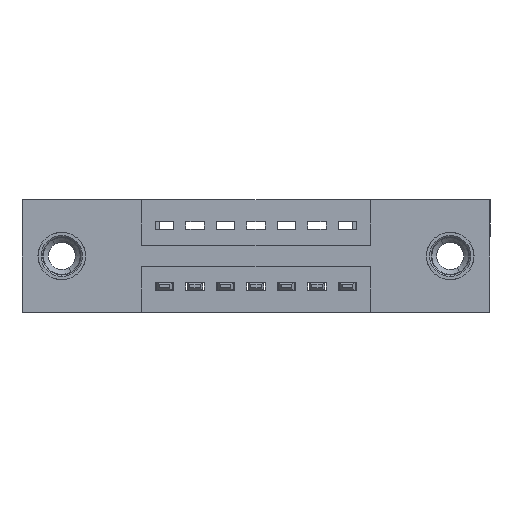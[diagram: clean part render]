
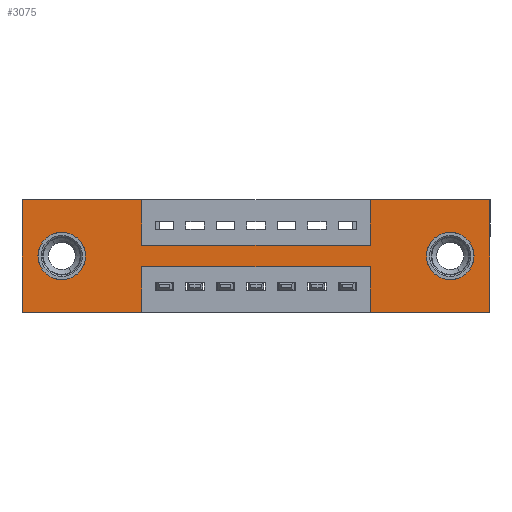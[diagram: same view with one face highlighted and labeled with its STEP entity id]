
A CAD part, front view. The second image highlights one B-rep face of the part: STEP entity #3075.
In plain terms, the highlighted planar face has unit normal (0, -1, 0).
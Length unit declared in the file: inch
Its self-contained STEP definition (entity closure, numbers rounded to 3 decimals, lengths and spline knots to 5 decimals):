
#88 = ORIENTED_EDGE ( 'NONE', *, *, #14354, .F. ) ;
#173 = LINE ( 'NONE', #8126, #4193 ) ;
#216 = DIRECTION ( 'NONE',  ( 1., 0., 0. ) ) ;
#373 = EDGE_CURVE ( 'NONE', #1136, #7667, #10331, .T. ) ;
#400 = DIRECTION ( 'NONE',  ( 0., 0., 1. ) ) ;
#508 = VECTOR ( 'NONE', #2237, 39.37008 ) ;
#535 = ORIENTED_EDGE ( 'NONE', *, *, #14030, .F. ) ;
#603 = CARTESIAN_POINT ( 'NONE',  ( 0.13, 0., -0.107 ) ) ;
#662 = LINE ( 'NONE', #11751, #7004 ) ;
#675 = CIRCLE ( 'NONE', #14537, 0.078 ) ;
#698 = LINE ( 'NONE', #5026, #1076 ) ;
#1076 = VECTOR ( 'NONE', #11715, 39.37008 ) ;
#1115 = VERTEX_POINT ( 'NONE', #603 ) ;
#1120 = VERTEX_POINT ( 'NONE', #5004 ) ;
#1136 = VERTEX_POINT ( 'NONE', #11938 ) ;
#1206 = CARTESIAN_POINT ( 'NONE',  ( 0., 0., -0.37 ) ) ;
#1337 = DIRECTION ( 'NONE',  ( 0., 1., 0. ) ) ;
#1531 = VERTEX_POINT ( 'NONE', #8712 ) ;
#1568 = LINE ( 'NONE', #10457, #3683 ) ;
#1743 = VECTOR ( 'NONE', #14314, 39.37008 ) ;
#1926 = VERTEX_POINT ( 'NONE', #7405 ) ;
#1986 = VECTOR ( 'NONE', #4073, 39.37008 ) ;
#2203 = DIRECTION ( 'NONE',  ( 0., 1., 0. ) ) ;
#2237 = DIRECTION ( 'NONE',  ( 0., 0., 1. ) ) ;
#2255 = ORIENTED_EDGE ( 'NONE', *, *, #14520, .F. ) ;
#2292 = VERTEX_POINT ( 'NONE', #3463 ) ;
#2590 = DIRECTION ( 'NONE',  ( -1., 0., 0. ) ) ;
#2808 = EDGE_LOOP ( 'NONE', ( #3830, #8100 ) ) ;
#2957 = LINE ( 'NONE', #11916, #11040 ) ;
#3075 = ADVANCED_FACE ( 'NONE', ( #6961, #6422, #11164 ), #5661, .T. ) ;
#3146 = EDGE_CURVE ( 'NONE', #7567, #14070, #4483, .T. ) ;
#3203 = EDGE_LOOP ( 'NONE', ( #13448, #6760 ) ) ;
#3404 = AXIS2_PLACEMENT_3D ( 'NONE', #3678, #1337, #400 ) ;
#3463 = CARTESIAN_POINT ( 'NONE',  ( 0.3925, 0., -0.22 ) ) ;
#3465 = DIRECTION ( 'NONE',  ( 0., 0., -1. ) ) ;
#3678 = CARTESIAN_POINT ( 'NONE',  ( 0.13, 0., -0.185 ) ) ;
#3683 = VECTOR ( 'NONE', #4623, 39.37008 ) ;
#3793 = ORIENTED_EDGE ( 'NONE', *, *, #4448, .F. ) ;
#3830 = ORIENTED_EDGE ( 'NONE', *, *, #10777, .T. ) ;
#3854 = CARTESIAN_POINT ( 'NONE',  ( 1.535, 0., -0.37 ) ) ;
#3884 = VERTEX_POINT ( 'NONE', #12785 ) ;
#3994 = DIRECTION ( 'NONE',  ( 0., 0., -1. ) ) ;
#4073 = DIRECTION ( 'NONE',  ( 0., 0., 1. ) ) ;
#4087 = DIRECTION ( 'NONE',  ( 0., 0., 1. ) ) ;
#4193 = VECTOR ( 'NONE', #2590, 39.37008 ) ;
#4389 = ORIENTED_EDGE ( 'NONE', *, *, #5117, .F. ) ;
#4448 = EDGE_CURVE ( 'NONE', #14070, #7242, #4953, .T. ) ;
#4483 = LINE ( 'NONE', #5605, #14157 ) ;
#4623 = DIRECTION ( 'NONE',  ( -1., 0., 0. ) ) ;
#4865 = CIRCLE ( 'NONE', #11131, 0.078 ) ;
#4953 = LINE ( 'NONE', #6335, #1986 ) ;
#5004 = CARTESIAN_POINT ( 'NONE',  ( 0., 0., -0.37 ) ) ;
#5026 = CARTESIAN_POINT ( 'NONE',  ( 0.3925, 0., -0.15 ) ) ;
#5117 = EDGE_CURVE ( 'NONE', #10800, #1926, #5188, .T. ) ;
#5173 = DIRECTION ( 'NONE',  ( 0., 0., 1. ) ) ;
#5188 = LINE ( 'NONE', #11372, #7318 ) ;
#5243 = CARTESIAN_POINT ( 'NONE',  ( 0., 0., 0. ) ) ;
#5605 = CARTESIAN_POINT ( 'NONE',  ( 0., 0., -0.37 ) ) ;
#5608 = VECTOR ( 'NONE', #6076, 39.37008 ) ;
#5661 = PLANE ( 'NONE',  #10589 ) ;
#6037 = CARTESIAN_POINT ( 'NONE',  ( 0.3925, 0., -0.37 ) ) ;
#6076 = DIRECTION ( 'NONE',  ( 0., 0., -1. ) ) ;
#6197 = DIRECTION ( 'NONE',  ( 0., 0., -1. ) ) ;
#6285 = ORIENTED_EDGE ( 'NONE', *, *, #9019, .F. ) ;
#6335 = CARTESIAN_POINT ( 'NONE',  ( 1.1425, 0., -0.37 ) ) ;
#6422 = FACE_BOUND ( 'NONE', #3203, .T. ) ;
#6444 = CARTESIAN_POINT ( 'NONE',  ( 1.1425, 0., -0.37 ) ) ;
#6685 = VECTOR ( 'NONE', #216, 39.37008 ) ;
#6760 = ORIENTED_EDGE ( 'NONE', *, *, #11376, .T. ) ;
#6806 = ORIENTED_EDGE ( 'NONE', *, *, #3146, .F. ) ;
#6824 = ORIENTED_EDGE ( 'NONE', *, *, #11123, .F. ) ;
#6961 = FACE_BOUND ( 'NONE', #2808, .T. ) ;
#7004 = VECTOR ( 'NONE', #6197, 39.37008 ) ;
#7124 = CARTESIAN_POINT ( 'NONE',  ( 1.535, 0., 0. ) ) ;
#7242 = VERTEX_POINT ( 'NONE', #14444 ) ;
#7318 = VECTOR ( 'NONE', #13600, 39.37008 ) ;
#7405 = CARTESIAN_POINT ( 'NONE',  ( 0.3925, 0., -0.15 ) ) ;
#7491 = CARTESIAN_POINT ( 'NONE',  ( 0.3925, 0., 0. ) ) ;
#7567 = VERTEX_POINT ( 'NONE', #3854 ) ;
#7625 = DIRECTION ( 'NONE',  ( 0., 1., 0. ) ) ;
#7667 = VERTEX_POINT ( 'NONE', #11470 ) ;
#7814 = DIRECTION ( 'NONE',  ( 0., -1., 0. ) ) ;
#7921 = CIRCLE ( 'NONE', #10911, 0.078 ) ;
#7998 = CARTESIAN_POINT ( 'NONE',  ( 0., 0., 0. ) ) ;
#8100 = ORIENTED_EDGE ( 'NONE', *, *, #8339, .T. ) ;
#8126 = CARTESIAN_POINT ( 'NONE',  ( 0., 0., -0.37 ) ) ;
#8339 = EDGE_CURVE ( 'NONE', #3884, #9829, #7921, .T. ) ;
#8712 = CARTESIAN_POINT ( 'NONE',  ( 0., 0., 0. ) ) ;
#8922 = EDGE_CURVE ( 'NONE', #1115, #9360, #11775, .T. ) ;
#8928 = ORIENTED_EDGE ( 'NONE', *, *, #14249, .F. ) ;
#9019 = EDGE_CURVE ( 'NONE', #1926, #1136, #698, .T. ) ;
#9246 = DIRECTION ( 'NONE',  ( 0., 1., 0. ) ) ;
#9307 = LINE ( 'NONE', #7998, #6685 ) ;
#9360 = VERTEX_POINT ( 'NONE', #10683 ) ;
#9829 = VERTEX_POINT ( 'NONE', #13728 ) ;
#9953 = VERTEX_POINT ( 'NONE', #6037 ) ;
#10331 = LINE ( 'NONE', #12354, #508 ) ;
#10396 = EDGE_CURVE ( 'NONE', #9953, #1120, #173, .T. ) ;
#10457 = CARTESIAN_POINT ( 'NONE',  ( 0.3925, 0., -0.22 ) ) ;
#10589 = AXIS2_PLACEMENT_3D ( 'NONE', #1206, #7814, #3465 ) ;
#10623 = CARTESIAN_POINT ( 'NONE',  ( 1.535, 0., 0. ) ) ;
#10683 = CARTESIAN_POINT ( 'NONE',  ( 0.13, 0., -0.263 ) ) ;
#10777 = EDGE_CURVE ( 'NONE', #9829, #3884, #675, .T. ) ;
#10800 = VERTEX_POINT ( 'NONE', #7491 ) ;
#10814 = CARTESIAN_POINT ( 'NONE',  ( 1.405, 0., -0.185 ) ) ;
#10911 = AXIS2_PLACEMENT_3D ( 'NONE', #11167, #9246, #12641 ) ;
#11040 = VECTOR ( 'NONE', #5173, 39.37008 ) ;
#11123 = EDGE_CURVE ( 'NONE', #2292, #9953, #662, .T. ) ;
#11131 = AXIS2_PLACEMENT_3D ( 'NONE', #14370, #7625, #4087 ) ;
#11164 = FACE_OUTER_BOUND ( 'NONE', #11595, .T. ) ;
#11167 = CARTESIAN_POINT ( 'NONE',  ( 1.405, 0., -0.185 ) ) ;
#11257 = LINE ( 'NONE', #5243, #1743 ) ;
#11372 = CARTESIAN_POINT ( 'NONE',  ( 0.3925, 0., 0. ) ) ;
#11376 = EDGE_CURVE ( 'NONE', #9360, #1115, #4865, .T. ) ;
#11470 = CARTESIAN_POINT ( 'NONE',  ( 1.1425, 0., 0. ) ) ;
#11595 = EDGE_LOOP ( 'NONE', ( #6824, #11834, #3793, #6806, #88, #8928, #12109, #6285, #4389, #535, #2255, #14294 ) ) ;
#11715 = DIRECTION ( 'NONE',  ( 1., 0., 0. ) ) ;
#11751 = CARTESIAN_POINT ( 'NONE',  ( 0.3925, 0., -0.37 ) ) ;
#11775 = CIRCLE ( 'NONE', #3404, 0.078 ) ;
#11834 = ORIENTED_EDGE ( 'NONE', *, *, #14268, .F. ) ;
#11916 = CARTESIAN_POINT ( 'NONE',  ( 0., 0., 0. ) ) ;
#11938 = CARTESIAN_POINT ( 'NONE',  ( 1.1425, 0., -0.15 ) ) ;
#12109 = ORIENTED_EDGE ( 'NONE', *, *, #373, .F. ) ;
#12354 = CARTESIAN_POINT ( 'NONE',  ( 1.1425, 0., 0. ) ) ;
#12641 = DIRECTION ( 'NONE',  ( 0., 0., -1. ) ) ;
#12785 = CARTESIAN_POINT ( 'NONE',  ( 1.405, 0., -0.263 ) ) ;
#13186 = VERTEX_POINT ( 'NONE', #10623 ) ;
#13448 = ORIENTED_EDGE ( 'NONE', *, *, #8922, .T. ) ;
#13483 = DIRECTION ( 'NONE',  ( -1., 0., 0. ) ) ;
#13600 = DIRECTION ( 'NONE',  ( 0., 0., -1. ) ) ;
#13728 = CARTESIAN_POINT ( 'NONE',  ( 1.405, 0., -0.107 ) ) ;
#13899 = LINE ( 'NONE', #7124, #5608 ) ;
#14030 = EDGE_CURVE ( 'NONE', #1531, #10800, #11257, .T. ) ;
#14070 = VERTEX_POINT ( 'NONE', #6444 ) ;
#14157 = VECTOR ( 'NONE', #13483, 39.37008 ) ;
#14249 = EDGE_CURVE ( 'NONE', #7667, #13186, #9307, .T. ) ;
#14268 = EDGE_CURVE ( 'NONE', #7242, #2292, #1568, .T. ) ;
#14294 = ORIENTED_EDGE ( 'NONE', *, *, #10396, .F. ) ;
#14314 = DIRECTION ( 'NONE',  ( 1., 0., 0. ) ) ;
#14354 = EDGE_CURVE ( 'NONE', #13186, #7567, #13899, .T. ) ;
#14370 = CARTESIAN_POINT ( 'NONE',  ( 0.13, 0., -0.185 ) ) ;
#14444 = CARTESIAN_POINT ( 'NONE',  ( 1.1425, 0., -0.22 ) ) ;
#14520 = EDGE_CURVE ( 'NONE', #1120, #1531, #2957, .T. ) ;
#14537 = AXIS2_PLACEMENT_3D ( 'NONE', #10814, #2203, #3994 ) ;
